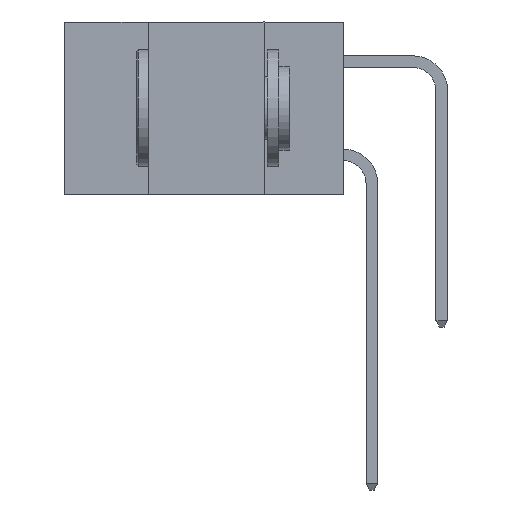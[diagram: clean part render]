
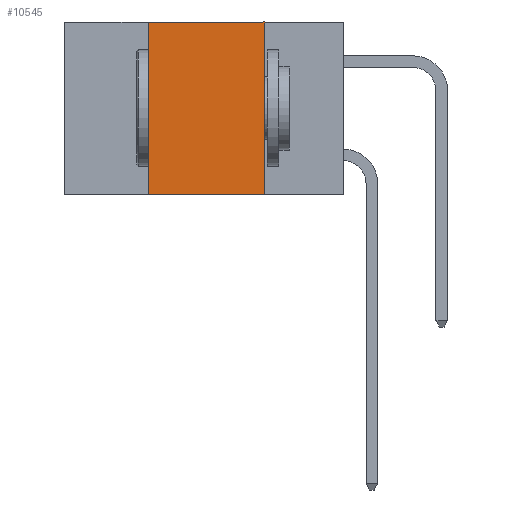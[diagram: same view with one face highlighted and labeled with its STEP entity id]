
A CAD part, left-side view. The second image highlights one B-rep face of the part: STEP entity #10545.
In plain terms, the highlighted planar face has unit normal (-1, 0, 0).
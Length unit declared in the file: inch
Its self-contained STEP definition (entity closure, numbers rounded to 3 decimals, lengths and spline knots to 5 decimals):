
#759 = VECTOR ( 'NONE', #25067, 39.37008 ) ;
#840 = LINE ( 'NONE', #19216, #11134 ) ;
#2036 = PLANE ( 'NONE',  #19075 ) ;
#4353 = EDGE_CURVE ( 'NONE', #11190, #6950, #14018, .T. ) ;
#6950 = VERTEX_POINT ( 'NONE', #11041 ) ;
#8234 = CARTESIAN_POINT ( 'NONE',  ( 0., 0.6, 0. ) ) ;
#9258 = CARTESIAN_POINT ( 'NONE',  ( 0., 0.17, -0.37 ) ) ;
#10312 = DIRECTION ( 'NONE',  ( 0., 0., -1. ) ) ;
#10545 = ADVANCED_FACE ( 'NONE', ( #25974 ), #2036, .F. ) ;
#10866 = CARTESIAN_POINT ( 'NONE',  ( 0., 0.42, -0.37 ) ) ;
#11041 = CARTESIAN_POINT ( 'NONE',  ( 0., 0.17, 0. ) ) ;
#11134 = VECTOR ( 'NONE', #21287, 39.37008 ) ;
#11190 = VERTEX_POINT ( 'NONE', #24479 ) ;
#12932 = DIRECTION ( 'NONE',  ( 0., 0., 1. ) ) ;
#12969 = VERTEX_POINT ( 'NONE', #16515 ) ;
#13703 = LINE ( 'NONE', #10866, #17876 ) ;
#14018 = LINE ( 'NONE', #16497, #24308 ) ;
#16368 = DIRECTION ( 'NONE',  ( 0., -1., 0. ) ) ;
#16497 = CARTESIAN_POINT ( 'NONE',  ( 0., 0.6, 0. ) ) ;
#16515 = CARTESIAN_POINT ( 'NONE',  ( 0., 0.42, -0.37 ) ) ;
#17876 = VECTOR ( 'NONE', #12932, 39.37008 ) ;
#19075 = AXIS2_PLACEMENT_3D ( 'NONE', #8234, #22635, #10312 ) ;
#19216 = CARTESIAN_POINT ( 'NONE',  ( 0., 0.17, -0.37 ) ) ;
#21287 = DIRECTION ( 'NONE',  ( 0., 0., -1. ) ) ;
#21368 = VERTEX_POINT ( 'NONE', #9258 ) ;
#21649 = EDGE_LOOP ( 'NONE', ( #23437, #26446, #23866, #24089 ) ) ;
#22631 = LINE ( 'NONE', #23037, #759 ) ;
#22635 = DIRECTION ( 'NONE',  ( 1., 0., 0. ) ) ;
#23037 = CARTESIAN_POINT ( 'NONE',  ( 0., 0.6, -0.37 ) ) ;
#23437 = ORIENTED_EDGE ( 'NONE', *, *, #24405, .F. ) ;
#23866 = ORIENTED_EDGE ( 'NONE', *, *, #24368, .F. ) ;
#24089 = ORIENTED_EDGE ( 'NONE', *, *, #25727, .T. ) ;
#24308 = VECTOR ( 'NONE', #16368, 39.37008 ) ;
#24368 = EDGE_CURVE ( 'NONE', #12969, #11190, #13703, .T. ) ;
#24405 = EDGE_CURVE ( 'NONE', #6950, #21368, #840, .T. ) ;
#24479 = CARTESIAN_POINT ( 'NONE',  ( 0., 0.42, 0. ) ) ;
#25067 = DIRECTION ( 'NONE',  ( 0., -1., 0. ) ) ;
#25727 = EDGE_CURVE ( 'NONE', #12969, #21368, #22631, .T. ) ;
#25974 = FACE_OUTER_BOUND ( 'NONE', #21649, .T. ) ;
#26446 = ORIENTED_EDGE ( 'NONE', *, *, #4353, .F. ) ;
